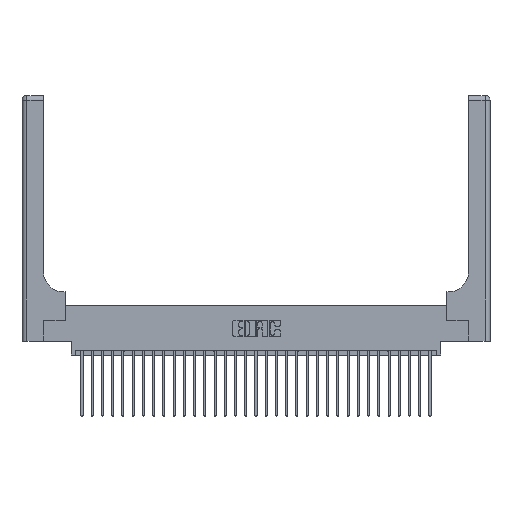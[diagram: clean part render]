
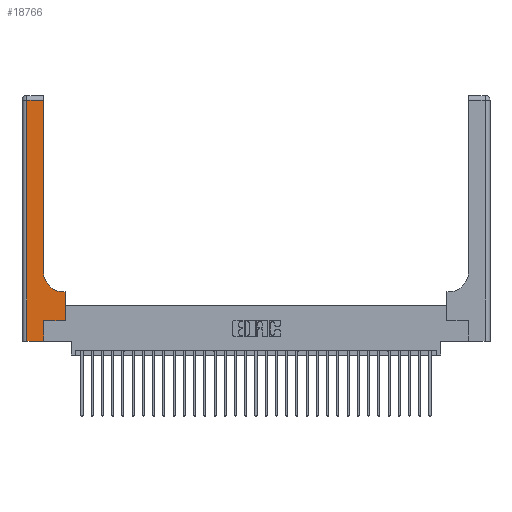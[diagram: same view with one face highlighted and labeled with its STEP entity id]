
A CAD part, top view. The second image highlights one B-rep face of the part: STEP entity #18766.
In plain terms, the highlighted planar face has unit normal (0, 0, 1).
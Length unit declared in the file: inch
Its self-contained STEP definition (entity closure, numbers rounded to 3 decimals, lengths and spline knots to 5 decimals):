
#230 = VECTOR ( 'NONE', #26394, 39.37008 ) ;
#778 = ORIENTED_EDGE ( 'NONE', *, *, #26462, .T. ) ;
#886 = AXIS2_PLACEMENT_3D ( 'NONE', #24962, #11554, #27200 ) ;
#1940 = DIRECTION ( 'NONE',  ( 0., 1., 0. ) ) ;
#2303 = DIRECTION ( 'NONE',  ( -1., 0., 0. ) ) ;
#2431 = LINE ( 'NONE', #26646, #13804 ) ;
#2555 = CARTESIAN_POINT ( 'NONE',  ( 0.26, 0.6, 0.37 ) ) ;
#2694 = EDGE_CURVE ( 'NONE', #25053, #9593, #28485, .T. ) ;
#3225 = AXIS2_PLACEMENT_3D ( 'NONE', #4464, #13594, #2303 ) ;
#3439 = EDGE_CURVE ( 'NONE', #26404, #25053, #15553, .T. ) ;
#4464 = CARTESIAN_POINT ( 'NONE',  ( 0., 3., 0.37 ) ) ;
#4554 = CARTESIAN_POINT ( 'NONE',  ( 0.265, 0.25, 0.37 ) ) ;
#4843 = CARTESIAN_POINT ( 'NONE',  ( 0.528, 0.6, 0.37 ) ) ;
#5484 = FACE_OUTER_BOUND ( 'NONE', #17783, .T. ) ;
#5734 = LINE ( 'NONE', #6229, #28920 ) ;
#6229 = CARTESIAN_POINT ( 'NONE',  ( 0., 0., 0.37 ) ) ;
#6246 = LINE ( 'NONE', #19719, #230 ) ;
#6771 = CARTESIAN_POINT ( 'NONE',  ( 0.06, 2.94, 0.37 ) ) ;
#6786 = CARTESIAN_POINT ( 'NONE',  ( 0.528, 0.25, 0.37 ) ) ;
#7293 = CARTESIAN_POINT ( 'NONE',  ( 0.26, 3., 0.37 ) ) ;
#8027 = CARTESIAN_POINT ( 'NONE',  ( 0.06, 3., 0.37 ) ) ;
#8175 = VERTEX_POINT ( 'NONE', #6786 ) ;
#8608 = VECTOR ( 'NONE', #8643, 39.37008 ) ;
#8643 = DIRECTION ( 'NONE',  ( 0., 1., 0. ) ) ;
#8844 = CARTESIAN_POINT ( 'NONE',  ( 0.06, 0., 0.37 ) ) ;
#8951 = ORIENTED_EDGE ( 'NONE', *, *, #22943, .T. ) ;
#9419 = DIRECTION ( 'NONE',  ( -1., 0., 0. ) ) ;
#9557 = ORIENTED_EDGE ( 'NONE', *, *, #3439, .T. ) ;
#9593 = VERTEX_POINT ( 'NONE', #25099 ) ;
#10758 = VERTEX_POINT ( 'NONE', #8844 ) ;
#11313 = CARTESIAN_POINT ( 'NONE',  ( 0.265, 0.25, 0.37 ) ) ;
#11554 = DIRECTION ( 'NONE',  ( 0., 0., -1. ) ) ;
#12854 = ORIENTED_EDGE ( 'NONE', *, *, #24414, .T. ) ;
#13462 = ORIENTED_EDGE ( 'NONE', *, *, #14487, .T. ) ;
#13594 = DIRECTION ( 'NONE',  ( 0., 0., -1. ) ) ;
#13804 = VECTOR ( 'NONE', #1940, 39.37008 ) ;
#14487 = EDGE_CURVE ( 'NONE', #8175, #26404, #25806, .T. ) ;
#14851 = VECTOR ( 'NONE', #15988, 39.37008 ) ;
#15050 = EDGE_CURVE ( 'NONE', #10758, #16620, #5734, .T. ) ;
#15553 = LINE ( 'NONE', #2555, #20810 ) ;
#15945 = LINE ( 'NONE', #8027, #24984 ) ;
#15988 = DIRECTION ( 'NONE',  ( 1., 0., 0. ) ) ;
#16316 = VERTEX_POINT ( 'NONE', #17277 ) ;
#16457 = DIRECTION ( 'NONE',  ( 0., 1., 0. ) ) ;
#16620 = VERTEX_POINT ( 'NONE', #18256 ) ;
#17164 = DIRECTION ( 'NONE',  ( 0., -1., 0. ) ) ;
#17277 = CARTESIAN_POINT ( 'NONE',  ( 0.26, 2.94, 0.37 ) ) ;
#17783 = EDGE_LOOP ( 'NONE', ( #778, #12854, #8951, #20965, #17829, #23723, #13462, #9557, #21556 ) ) ;
#17829 = ORIENTED_EDGE ( 'NONE', *, *, #28503, .T. ) ;
#18192 = LINE ( 'NONE', #7293, #18887 ) ;
#18256 = CARTESIAN_POINT ( 'NONE',  ( 0.265, 0., 0.37 ) ) ;
#18766 = ADVANCED_FACE ( 'NONE', ( #5484 ), #26975, .F. ) ;
#18887 = VECTOR ( 'NONE', #16457, 39.37008 ) ;
#19719 = CARTESIAN_POINT ( 'NONE',  ( 0., 2.94, 0.37 ) ) ;
#19906 = CARTESIAN_POINT ( 'NONE',  ( 0.528, 0.25, 0.37 ) ) ;
#19966 = CARTESIAN_POINT ( 'NONE',  ( 0.51, 0.6, 0.37 ) ) ;
#20676 = VERTEX_POINT ( 'NONE', #6771 ) ;
#20810 = VECTOR ( 'NONE', #9419, 39.37008 ) ;
#20837 = LINE ( 'NONE', #4554, #14851 ) ;
#20965 = ORIENTED_EDGE ( 'NONE', *, *, #15050, .T. ) ;
#21556 = ORIENTED_EDGE ( 'NONE', *, *, #2694, .T. ) ;
#22943 = EDGE_CURVE ( 'NONE', #20676, #10758, #15945, .T. ) ;
#23723 = ORIENTED_EDGE ( 'NONE', *, *, #28692, .T. ) ;
#24229 = DIRECTION ( 'NONE',  ( 1., 0., 0. ) ) ;
#24414 = EDGE_CURVE ( 'NONE', #16316, #20676, #6246, .T. ) ;
#24962 = CARTESIAN_POINT ( 'NONE',  ( 0.51, 0.85, 0.37 ) ) ;
#24984 = VECTOR ( 'NONE', #17164, 39.37008 ) ;
#25053 = VERTEX_POINT ( 'NONE', #19966 ) ;
#25099 = CARTESIAN_POINT ( 'NONE',  ( 0.26, 0.85, 0.37 ) ) ;
#25806 = LINE ( 'NONE', #19906, #8608 ) ;
#26394 = DIRECTION ( 'NONE',  ( -1., 0., 0. ) ) ;
#26404 = VERTEX_POINT ( 'NONE', #4843 ) ;
#26462 = EDGE_CURVE ( 'NONE', #9593, #16316, #18192, .T. ) ;
#26646 = CARTESIAN_POINT ( 'NONE',  ( 0.265, 0., 0.37 ) ) ;
#26975 = PLANE ( 'NONE',  #3225 ) ;
#27200 = DIRECTION ( 'NONE',  ( 1., 0., 0. ) ) ;
#28485 = CIRCLE ( 'NONE', #886, 0.25 ) ;
#28503 = EDGE_CURVE ( 'NONE', #16620, #28667, #2431, .T. ) ;
#28667 = VERTEX_POINT ( 'NONE', #11313 ) ;
#28692 = EDGE_CURVE ( 'NONE', #28667, #8175, #20837, .T. ) ;
#28920 = VECTOR ( 'NONE', #24229, 39.37008 ) ;
